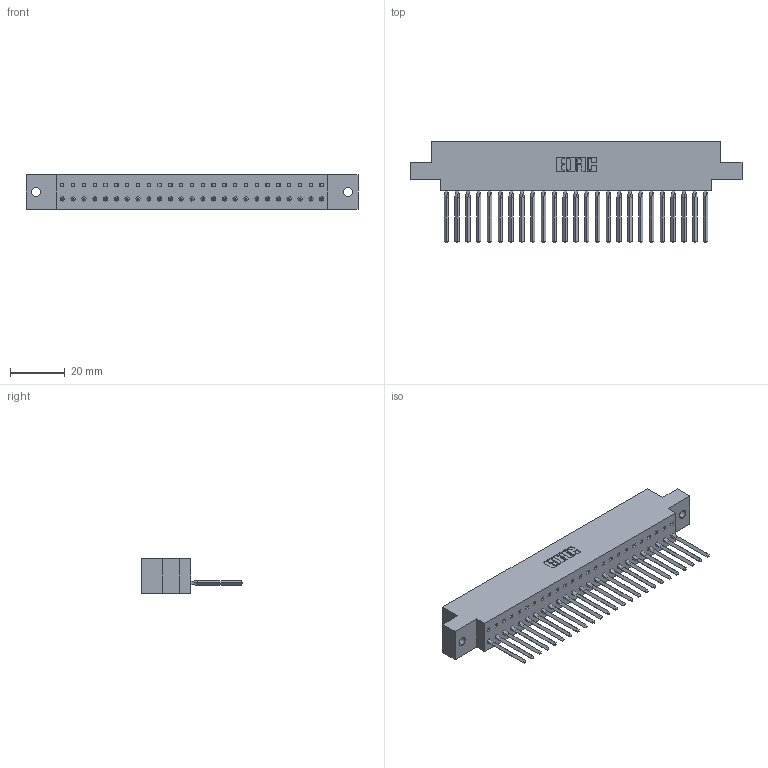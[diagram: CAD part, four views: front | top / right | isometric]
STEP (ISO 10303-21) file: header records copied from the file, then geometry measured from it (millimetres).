
FILE_DESCRIPTION (( 'STEP AP203' ), '1' );
FILE_NAME ('317-025-541-602.STEP', '2020-02-27T18:28:39', ( '' ), ( '' ), 'SwSTEP 2.0', 'SolidWorks 2016', '' );
FILE_SCHEMA (( 'CONFIG_CONTROL_DESIGN' ));
Length unit declared in the file: inch
Products named in the file (3): 317-025-541-602; 317-290-002_541; 317 Part_.144 Dia
Assembly tree (26 placements, depth 2):
  317-025-541-602
    317 Part_.144 Dia
    317-290-002_541  x25
Bounding box: 121.77 x 37.34 x 12.7 mm (x, y, z)
Volume: 19187.2 mm3; surface area: 26279.5 mm2
Topology: 26 solids, 26 shells, 3902 faces, 11125 edges, 7232 vertices
Faces by surface type: plane 3158, cylinder 644, bspline 100
Entity records: 39260 total; most frequent: CARTESIAN_POINT 7612, ORIENTED_EDGE 6890, DIRECTION 5647, EDGE_CURVE 3445, VECTOR 3081, LINE 3081, VERTEX_POINT 2288, AXIS2_PLACEMENT_3D 1283
